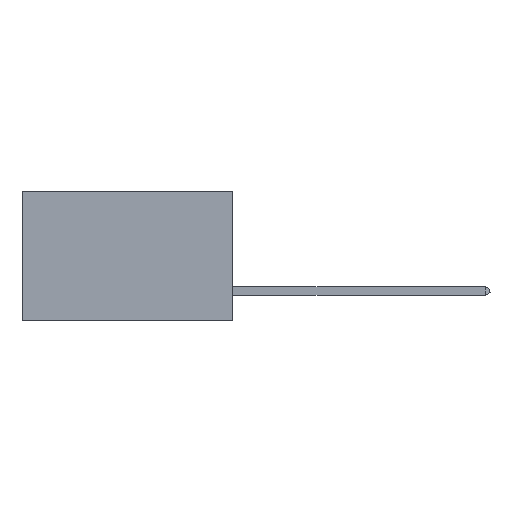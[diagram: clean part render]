
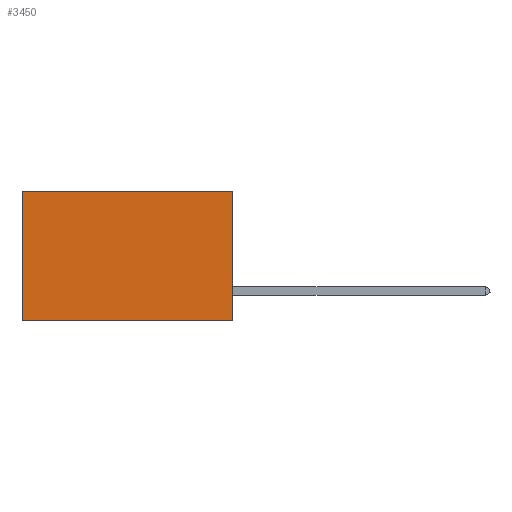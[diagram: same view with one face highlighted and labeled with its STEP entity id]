
A CAD part, left-side view. The second image highlights one B-rep face of the part: STEP entity #3450.
In plain terms, the highlighted planar face has unit normal (-1, 0, 0).
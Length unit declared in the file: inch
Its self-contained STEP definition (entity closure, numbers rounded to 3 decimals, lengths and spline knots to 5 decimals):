
#153 = ORIENTED_EDGE ( 'NONE', *, *, #8088, .F. ) ;
#1937 = AXIS2_PLACEMENT_3D ( 'NONE', #2885, #20582, #45413 ) ;
#2091 = VERTEX_POINT ( 'NONE', #8442 ) ;
#2628 = DIRECTION ( 'NONE',  ( 0., 1., 0. ) ) ;
#2885 = CARTESIAN_POINT ( 'NONE',  ( 0.2875, 0., 0. ) ) ;
#3292 = VECTOR ( 'NONE', #2628, 39.37008 ) ;
#3450 = ADVANCED_FACE ( 'NONE', ( #21982 ), #42173, .F. ) ;
#4630 = LINE ( 'NONE', #12339, #45327 ) ;
#5163 = ORIENTED_EDGE ( 'NONE', *, *, #45850, .T. ) ;
#7808 = DIRECTION ( 'NONE',  ( 0., 0., -1. ) ) ;
#8008 = ORIENTED_EDGE ( 'NONE', *, *, #30553, .T. ) ;
#8088 = EDGE_CURVE ( 'NONE', #43310, #2091, #4630, .T. ) ;
#8154 = DIRECTION ( 'NONE',  ( 0., 1., 0. ) ) ;
#8442 = CARTESIAN_POINT ( 'NONE',  ( 0.2875, 0., -0.37 ) ) ;
#8550 = DIRECTION ( 'NONE',  ( 0., 0., -1. ) ) ;
#11453 = CARTESIAN_POINT ( 'NONE',  ( 0.2875, 0., -0.37 ) ) ;
#11828 = CARTESIAN_POINT ( 'NONE',  ( 0.2875, 0.6, -0.37 ) ) ;
#12021 = EDGE_LOOP ( 'NONE', ( #8008, #35177, #153, #5163 ) ) ;
#12339 = CARTESIAN_POINT ( 'NONE',  ( 0.2875, 0., 0. ) ) ;
#19946 = EDGE_CURVE ( 'NONE', #2091, #29502, #43634, .T. ) ;
#19960 = CARTESIAN_POINT ( 'NONE',  ( 0.2875, 0., 0. ) ) ;
#20582 = DIRECTION ( 'NONE',  ( 1., 0., 0. ) ) ;
#21982 = FACE_OUTER_BOUND ( 'NONE', #12021, .T. ) ;
#22083 = CARTESIAN_POINT ( 'NONE',  ( 0.2875, 0.6, 0. ) ) ;
#24378 = CARTESIAN_POINT ( 'NONE',  ( 0.2875, 0., 0. ) ) ;
#24692 = CARTESIAN_POINT ( 'NONE',  ( 0.2875, 0.6, 0. ) ) ;
#29502 = VERTEX_POINT ( 'NONE', #11828 ) ;
#30553 = EDGE_CURVE ( 'NONE', #36790, #29502, #43594, .T. ) ;
#35177 = ORIENTED_EDGE ( 'NONE', *, *, #19946, .F. ) ;
#35685 = LINE ( 'NONE', #24378, #3292 ) ;
#35869 = VECTOR ( 'NONE', #7808, 39.37008 ) ;
#36790 = VERTEX_POINT ( 'NONE', #24692 ) ;
#42173 = PLANE ( 'NONE',  #1937 ) ;
#43310 = VERTEX_POINT ( 'NONE', #19960 ) ;
#43594 = LINE ( 'NONE', #22083, #35869 ) ;
#43634 = LINE ( 'NONE', #11453, #44768 ) ;
#44768 = VECTOR ( 'NONE', #8154, 39.37008 ) ;
#45327 = VECTOR ( 'NONE', #8550, 39.37008 ) ;
#45413 = DIRECTION ( 'NONE',  ( 0., 0., -1. ) ) ;
#45850 = EDGE_CURVE ( 'NONE', #43310, #36790, #35685, .T. ) ;
